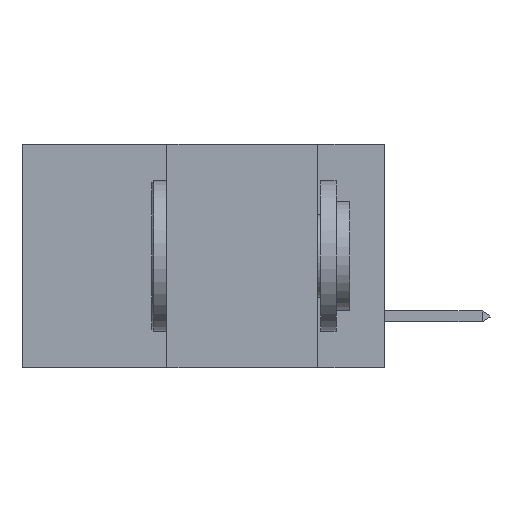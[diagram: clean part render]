
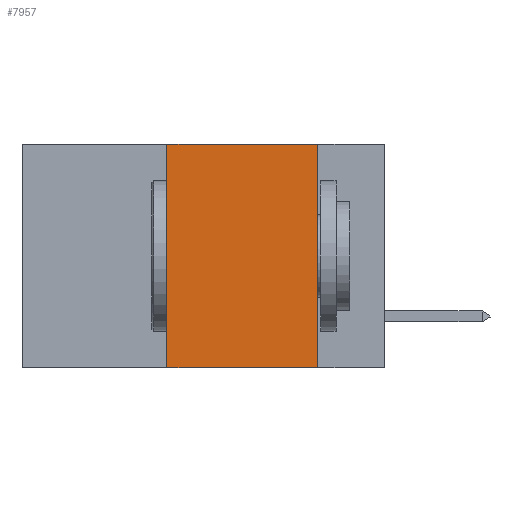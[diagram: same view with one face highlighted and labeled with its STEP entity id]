
A CAD part, left-side view. The second image highlights one B-rep face of the part: STEP entity #7957.
In plain terms, the highlighted planar face has unit normal (-1, 0, 0).
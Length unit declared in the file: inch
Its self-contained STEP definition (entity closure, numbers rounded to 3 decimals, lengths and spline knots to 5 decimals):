
#356 = DIRECTION ( 'NONE',  ( 1., 0., 0. ) ) ;
#660 = VERTEX_POINT ( 'NONE', #5391 ) ;
#757 = VERTEX_POINT ( 'NONE', #13654 ) ;
#848 = VERTEX_POINT ( 'NONE', #11450 ) ;
#1000 = EDGE_CURVE ( 'NONE', #660, #757, #2874, .T. ) ;
#1597 = CARTESIAN_POINT ( 'NONE',  ( 0., 0.6, -0.37 ) ) ;
#1673 = CARTESIAN_POINT ( 'NONE',  ( 0., 0.6, 0. ) ) ;
#1889 = DIRECTION ( 'NONE',  ( 0., -1., 0. ) ) ;
#1979 = CARTESIAN_POINT ( 'NONE',  ( 0., 0.6, 0. ) ) ;
#2554 = VECTOR ( 'NONE', #3581, 39.37008 ) ;
#2874 = LINE ( 'NONE', #9548, #3930 ) ;
#3581 = DIRECTION ( 'NONE',  ( 0., 0., -1. ) ) ;
#3930 = VECTOR ( 'NONE', #10662, 39.37008 ) ;
#4257 = EDGE_CURVE ( 'NONE', #757, #848, #8587, .T. ) ;
#4968 = DIRECTION ( 'NONE',  ( 0., -1., 0. ) ) ;
#5185 = AXIS2_PLACEMENT_3D ( 'NONE', #1673, #356, #13848 ) ;
#5391 = CARTESIAN_POINT ( 'NONE',  ( 0., 0.36, -0.37 ) ) ;
#5525 = EDGE_CURVE ( 'NONE', #848, #8762, #7661, .T. ) ;
#5572 = VECTOR ( 'NONE', #1889, 39.37008 ) ;
#5810 = CARTESIAN_POINT ( 'NONE',  ( 0., 0.11, 0. ) ) ;
#7016 = VECTOR ( 'NONE', #4968, 39.37008 ) ;
#7661 = LINE ( 'NONE', #5810, #2554 ) ;
#7957 = ADVANCED_FACE ( 'NONE', ( #7963 ), #12288, .F. ) ;
#7963 = FACE_OUTER_BOUND ( 'NONE', #14184, .T. ) ;
#8587 = LINE ( 'NONE', #1979, #5572 ) ;
#8762 = VERTEX_POINT ( 'NONE', #10494 ) ;
#9548 = CARTESIAN_POINT ( 'NONE',  ( 0., 0.36, 0. ) ) ;
#10485 = ORIENTED_EDGE ( 'NONE', *, *, #4257, .F. ) ;
#10494 = CARTESIAN_POINT ( 'NONE',  ( 0., 0.11, -0.37 ) ) ;
#10662 = DIRECTION ( 'NONE',  ( 0., 0., 1. ) ) ;
#11282 = EDGE_CURVE ( 'NONE', #660, #8762, #14041, .T. ) ;
#11450 = CARTESIAN_POINT ( 'NONE',  ( 0., 0.11, 0. ) ) ;
#11658 = ORIENTED_EDGE ( 'NONE', *, *, #1000, .F. ) ;
#12288 = PLANE ( 'NONE',  #5185 ) ;
#12790 = ORIENTED_EDGE ( 'NONE', *, *, #11282, .T. ) ;
#13654 = CARTESIAN_POINT ( 'NONE',  ( 0., 0.36, 0. ) ) ;
#13848 = DIRECTION ( 'NONE',  ( 0., 0., -1. ) ) ;
#14041 = LINE ( 'NONE', #1597, #7016 ) ;
#14184 = EDGE_LOOP ( 'NONE', ( #14403, #10485, #11658, #12790 ) ) ;
#14403 = ORIENTED_EDGE ( 'NONE', *, *, #5525, .F. ) ;
